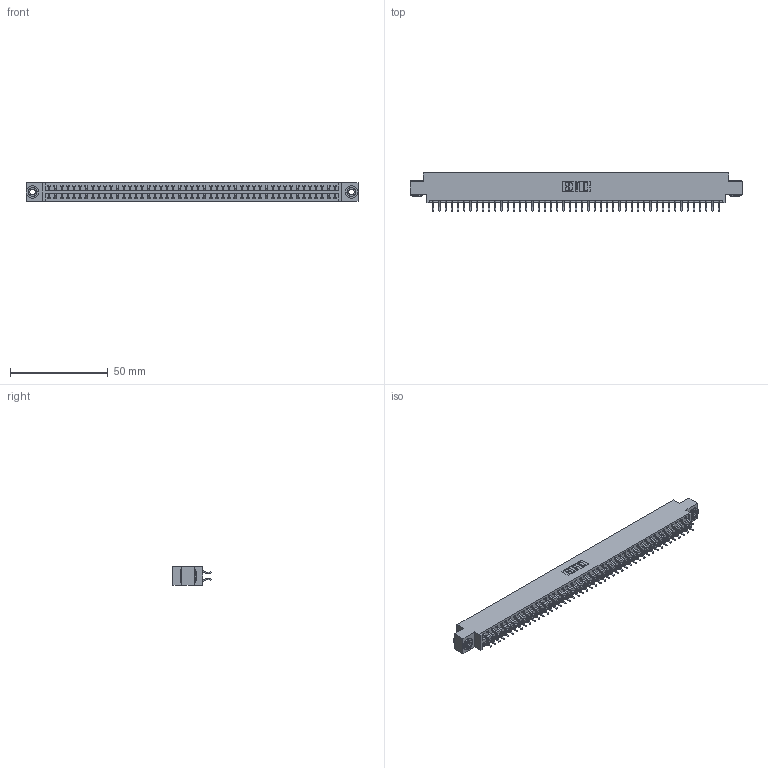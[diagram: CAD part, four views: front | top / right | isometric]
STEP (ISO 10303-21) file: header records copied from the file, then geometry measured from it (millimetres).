
FILE_DESCRIPTION (( 'STEP AP203' ), '1' );
FILE_NAME ('346-094-556-803.STEP', '2022-05-26T15:03:37', ( '' ), ( '' ), 'SwSTEP 2.0', 'SolidWorks 2020', '' );
FILE_SCHEMA (( 'CONFIG_CONTROL_DESIGN' ));
Length unit declared in the file: inch
Products named in the file (4): 345-250-002_345-250-002-102; 346 Part_0.170 Offset - 0.156 Dia-TH; 345-292-001_556 Tail; 346-094-556-803
Assembly tree (97 placements, depth 2):
  346-094-556-803
    346 Part_0.170 Offset - 0.156 Dia-TH
    345-292-001_556 Tail  x94
    345-250-002_345-250-002-102  x2
Bounding box: 169.8 x 19.57 x 9.4 mm (x, y, z)
Volume: 16439.3 mm3; surface area: 23016.6 mm2
Topology: 97 solids, 97 shells, 5630 faces, 16715 edges, 11014 vertices
Faces by surface type: plane 3770, cylinder 1852, cone 8
Entity records: 31418 total; most frequent: CARTESIAN_POINT 5169, ORIENTED_EDGE 5082, DIRECTION 4623, EDGE_CURVE 2541, LINE 2189, VECTOR 2189, VERTEX_POINT 1690, AXIS2_PLACEMENT_3D 1217
